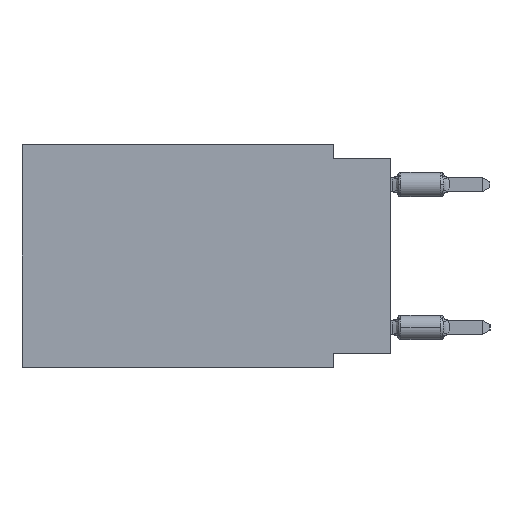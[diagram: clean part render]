
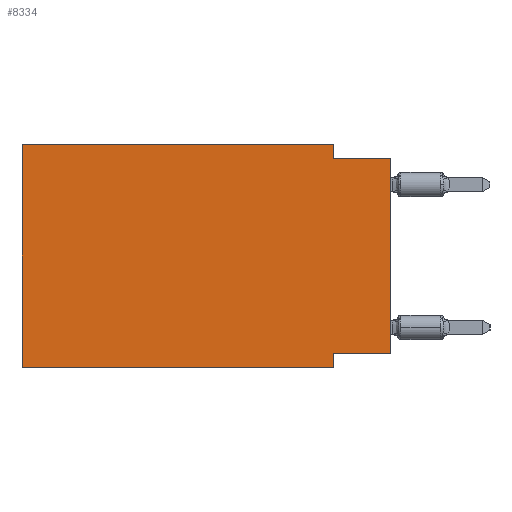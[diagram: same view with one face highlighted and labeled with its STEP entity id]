
A CAD part, left-side view. The second image highlights one B-rep face of the part: STEP entity #8334.
In plain terms, the highlighted planar face has unit normal (-1, 0, 0).
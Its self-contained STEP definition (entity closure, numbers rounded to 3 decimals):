
#340 = ORIENTED_EDGE ( 'NONE', *, *, #1962, .F. ) ;
#943 = CARTESIAN_POINT ( 'NONE',  ( 0., 0., -9.271 ) ) ;
#996 = VERTEX_POINT ( 'NONE', #5032 ) ;
#1066 = CARTESIAN_POINT ( 'NONE',  ( 0., 16.383, 0. ) ) ;
#1209 = CARTESIAN_POINT ( 'NONE',  ( 0., 16.383, 0. ) ) ;
#1234 = EDGE_CURVE ( 'NONE', #6939, #16439, #7970, .T. ) ;
#1418 = PLANE ( 'NONE',  #2511 ) ;
#1961 = EDGE_CURVE ( 'NONE', #996, #16439, #21236, .T. ) ;
#1962 = EDGE_CURVE ( 'NONE', #996, #4138, #4799, .T. ) ;
#2330 = EDGE_LOOP ( 'NONE', ( #4154, #13711, #17068, #20820, #340, #11512, #19490, #17278 ) ) ;
#2511 = AXIS2_PLACEMENT_3D ( 'NONE', #1209, #7907, #3077 ) ;
#2700 = LINE ( 'NONE', #943, #15051 ) ;
#3077 = DIRECTION ( 'NONE',  ( 0., 0., -1. ) ) ;
#4138 = VERTEX_POINT ( 'NONE', #15402 ) ;
#4154 = ORIENTED_EDGE ( 'NONE', *, *, #18192, .T. ) ;
#4799 = LINE ( 'NONE', #1066, #18519 ) ;
#4959 = CARTESIAN_POINT ( 'NONE',  ( 0., 2.54, -9.271 ) ) ;
#5032 = CARTESIAN_POINT ( 'NONE',  ( 0., 16.383, -9.906 ) ) ;
#5333 = LINE ( 'NONE', #15225, #19808 ) ;
#5376 = CARTESIAN_POINT ( 'NONE',  ( 0., 0., -9.271 ) ) ;
#6305 = LINE ( 'NONE', #16417, #8782 ) ;
#6337 = DIRECTION ( 'NONE',  ( 0., 0., 1. ) ) ;
#6753 = DIRECTION ( 'NONE',  ( 0., 0., 1. ) ) ;
#6939 = VERTEX_POINT ( 'NONE', #4959 ) ;
#7006 = VERTEX_POINT ( 'NONE', #17557 ) ;
#7008 = CARTESIAN_POINT ( 'NONE',  ( 0., 2.54, -9.906 ) ) ;
#7534 = EDGE_CURVE ( 'NONE', #4138, #7006, #6305, .T. ) ;
#7541 = CARTESIAN_POINT ( 'NONE',  ( 0., 2.54, -9.906 ) ) ;
#7632 = DIRECTION ( 'NONE',  ( 0., 1., 0. ) ) ;
#7907 = DIRECTION ( 'NONE',  ( 1., 0., 0. ) ) ;
#7970 = LINE ( 'NONE', #7541, #11304 ) ;
#8174 = CARTESIAN_POINT ( 'NONE',  ( 0., 0., -0.635 ) ) ;
#8334 = ADVANCED_FACE ( 'NONE', ( #16266 ), #1418, .F. ) ;
#8782 = VECTOR ( 'NONE', #15923, 1000. ) ;
#8811 = VECTOR ( 'NONE', #13153, 1000. ) ;
#9601 = DIRECTION ( 'NONE',  ( 0., 0., -1. ) ) ;
#10763 = VERTEX_POINT ( 'NONE', #8174 ) ;
#10896 = VECTOR ( 'NONE', #18129, 1000. ) ;
#11007 = CARTESIAN_POINT ( 'NONE',  ( 0., 2.54, 0. ) ) ;
#11134 = LINE ( 'NONE', #12638, #12784 ) ;
#11304 = VECTOR ( 'NONE', #9601, 1000. ) ;
#11512 = ORIENTED_EDGE ( 'NONE', *, *, #1961, .T. ) ;
#12638 = CARTESIAN_POINT ( 'NONE',  ( 0., 0., -0.635 ) ) ;
#12784 = VECTOR ( 'NONE', #21033, 1000. ) ;
#12840 = CARTESIAN_POINT ( 'NONE',  ( 0., 16.383, -9.906 ) ) ;
#13130 = VERTEX_POINT ( 'NONE', #5376 ) ;
#13153 = DIRECTION ( 'NONE',  ( 0., -1., 0. ) ) ;
#13711 = ORIENTED_EDGE ( 'NONE', *, *, #16635, .F. ) ;
#14859 = LINE ( 'NONE', #11007, #10896 ) ;
#15051 = VECTOR ( 'NONE', #7632, 1000. ) ;
#15225 = CARTESIAN_POINT ( 'NONE',  ( 0., 0., 0. ) ) ;
#15234 = CARTESIAN_POINT ( 'NONE',  ( 0., 2.54, -0.635 ) ) ;
#15402 = CARTESIAN_POINT ( 'NONE',  ( 0., 16.383, 0. ) ) ;
#15923 = DIRECTION ( 'NONE',  ( 0., -1., 0. ) ) ;
#16266 = FACE_OUTER_BOUND ( 'NONE', #2330, .T. ) ;
#16417 = CARTESIAN_POINT ( 'NONE',  ( 0., 16.383, 0. ) ) ;
#16439 = VERTEX_POINT ( 'NONE', #7008 ) ;
#16635 = EDGE_CURVE ( 'NONE', #16877, #10763, #11134, .T. ) ;
#16877 = VERTEX_POINT ( 'NONE', #15234 ) ;
#17068 = ORIENTED_EDGE ( 'NONE', *, *, #21287, .F. ) ;
#17278 = ORIENTED_EDGE ( 'NONE', *, *, #21315, .F. ) ;
#17557 = CARTESIAN_POINT ( 'NONE',  ( 0., 2.54, 0. ) ) ;
#18129 = DIRECTION ( 'NONE',  ( 0., 0., -1. ) ) ;
#18192 = EDGE_CURVE ( 'NONE', #13130, #10763, #5333, .T. ) ;
#18519 = VECTOR ( 'NONE', #6337, 1000. ) ;
#19490 = ORIENTED_EDGE ( 'NONE', *, *, #1234, .F. ) ;
#19808 = VECTOR ( 'NONE', #6753, 1000. ) ;
#20820 = ORIENTED_EDGE ( 'NONE', *, *, #7534, .F. ) ;
#21033 = DIRECTION ( 'NONE',  ( 0., -1., 0. ) ) ;
#21236 = LINE ( 'NONE', #12840, #8811 ) ;
#21287 = EDGE_CURVE ( 'NONE', #7006, #16877, #14859, .T. ) ;
#21315 = EDGE_CURVE ( 'NONE', #13130, #6939, #2700, .T. ) ;
